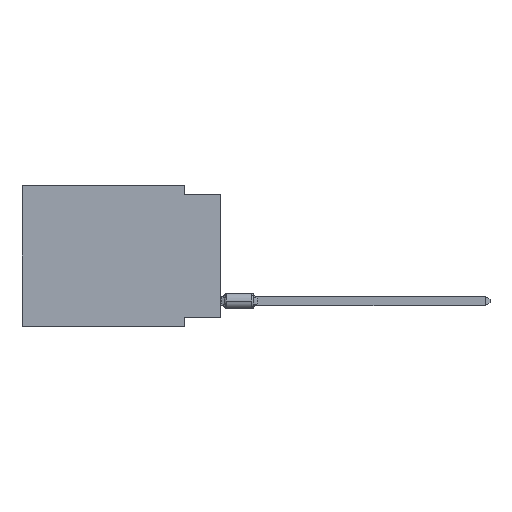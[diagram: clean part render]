
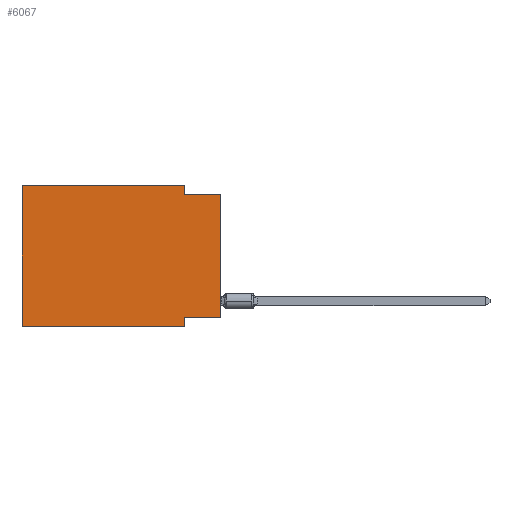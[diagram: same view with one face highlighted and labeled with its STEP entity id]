
A CAD part, left-side view. The second image highlights one B-rep face of the part: STEP entity #6067.
In plain terms, the highlighted planar face has unit normal (-1, 0, 0).
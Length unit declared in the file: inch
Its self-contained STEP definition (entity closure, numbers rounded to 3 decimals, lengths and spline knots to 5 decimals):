
#204 = VERTEX_POINT ( 'NONE', #6549 ) ;
#2309 = DIRECTION ( 'NONE',  ( 0., 0., -1. ) ) ;
#2672 = VERTEX_POINT ( 'NONE', #25112 ) ;
#3417 = VERTEX_POINT ( 'NONE', #29619 ) ;
#3538 = CARTESIAN_POINT ( 'NONE',  ( 0., 0., -0.025 ) ) ;
#3562 = VECTOR ( 'NONE', #2309, 39.37008 ) ;
#3690 = CARTESIAN_POINT ( 'NONE',  ( 0., 0., 0. ) ) ;
#3943 = CARTESIAN_POINT ( 'NONE',  ( 0., 0.1, 0. ) ) ;
#3959 = VECTOR ( 'NONE', #8955, 39.37008 ) ;
#4258 = ORIENTED_EDGE ( 'NONE', *, *, #20198, .F. ) ;
#4618 = EDGE_CURVE ( 'NONE', #204, #3417, #23734, .T. ) ;
#4672 = CARTESIAN_POINT ( 'NONE',  ( 0., 0.1, -0.39 ) ) ;
#5339 = LINE ( 'NONE', #34681, #6964 ) ;
#6067 = ADVANCED_FACE ( 'NONE', ( #21899 ), #22459, .F. ) ;
#6472 = VERTEX_POINT ( 'NONE', #13834 ) ;
#6549 = CARTESIAN_POINT ( 'NONE',  ( 0., 0.55, 0. ) ) ;
#6585 = VERTEX_POINT ( 'NONE', #14967 ) ;
#6964 = VECTOR ( 'NONE', #20259, 39.37008 ) ;
#8955 = DIRECTION ( 'NONE',  ( 0., 0., 1. ) ) ;
#9156 = DIRECTION ( 'NONE',  ( 0., -1., 0. ) ) ;
#9715 = DIRECTION ( 'NONE',  ( 0., -1., 0. ) ) ;
#9748 = VECTOR ( 'NONE', #9156, 39.37008 ) ;
#10490 = EDGE_CURVE ( 'NONE', #3417, #2672, #29848, .T. ) ;
#10832 = ORIENTED_EDGE ( 'NONE', *, *, #33181, .F. ) ;
#11297 = ORIENTED_EDGE ( 'NONE', *, *, #18778, .F. ) ;
#11999 = CARTESIAN_POINT ( 'NONE',  ( 0., 0.55, 0. ) ) ;
#12573 = LINE ( 'NONE', #3538, #19518 ) ;
#12607 = DIRECTION ( 'NONE',  ( 0., 0., -1. ) ) ;
#13574 = VECTOR ( 'NONE', #26691, 39.37008 ) ;
#13834 = CARTESIAN_POINT ( 'NONE',  ( 0., 0., -0.365 ) ) ;
#14967 = CARTESIAN_POINT ( 'NONE',  ( 0., 0.55, -0.39 ) ) ;
#15401 = LINE ( 'NONE', #35680, #36812 ) ;
#15549 = EDGE_LOOP ( 'NONE', ( #34981, #10832, #30154, #18344, #4258, #22154, #11297, #31808 ) ) ;
#17045 = CARTESIAN_POINT ( 'NONE',  ( 0., 0.1, -0.365 ) ) ;
#17069 = EDGE_CURVE ( 'NONE', #6585, #26470, #15401, .T. ) ;
#17406 = CARTESIAN_POINT ( 'NONE',  ( 0., 0.55, 0. ) ) ;
#17980 = LINE ( 'NONE', #17406, #13574 ) ;
#18344 = ORIENTED_EDGE ( 'NONE', *, *, #4618, .F. ) ;
#18778 = EDGE_CURVE ( 'NONE', #31019, #26470, #25176, .T. ) ;
#19518 = VECTOR ( 'NONE', #23936, 39.37008 ) ;
#20198 = EDGE_CURVE ( 'NONE', #6585, #204, #17980, .T. ) ;
#20259 = DIRECTION ( 'NONE',  ( 0., 1., 0. ) ) ;
#21899 = FACE_OUTER_BOUND ( 'NONE', #15549, .T. ) ;
#22090 = EDGE_CURVE ( 'NONE', #6472, #22195, #29604, .T. ) ;
#22154 = ORIENTED_EDGE ( 'NONE', *, *, #17069, .T. ) ;
#22195 = VERTEX_POINT ( 'NONE', #36598 ) ;
#22459 = PLANE ( 'NONE',  #24341 ) ;
#23734 = LINE ( 'NONE', #11999, #9748 ) ;
#23936 = DIRECTION ( 'NONE',  ( 0., -1., 0. ) ) ;
#24341 = AXIS2_PLACEMENT_3D ( 'NONE', #33463, #28519, #33837 ) ;
#25112 = CARTESIAN_POINT ( 'NONE',  ( 0., 0.1, -0.025 ) ) ;
#25176 = LINE ( 'NONE', #25354, #3562 ) ;
#25354 = CARTESIAN_POINT ( 'NONE',  ( 0., 0.1, -0.39 ) ) ;
#26470 = VERTEX_POINT ( 'NONE', #4672 ) ;
#26691 = DIRECTION ( 'NONE',  ( 0., 0., 1. ) ) ;
#28519 = DIRECTION ( 'NONE',  ( 1., 0., 0. ) ) ;
#29604 = LINE ( 'NONE', #3690, #3959 ) ;
#29619 = CARTESIAN_POINT ( 'NONE',  ( 0., 0.1, 0. ) ) ;
#29826 = VECTOR ( 'NONE', #12607, 39.37008 ) ;
#29848 = LINE ( 'NONE', #3943, #29826 ) ;
#30154 = ORIENTED_EDGE ( 'NONE', *, *, #10490, .F. ) ;
#31019 = VERTEX_POINT ( 'NONE', #17045 ) ;
#31808 = ORIENTED_EDGE ( 'NONE', *, *, #35087, .F. ) ;
#33181 = EDGE_CURVE ( 'NONE', #2672, #22195, #12573, .T. ) ;
#33463 = CARTESIAN_POINT ( 'NONE',  ( 0., 0.55, 0. ) ) ;
#33837 = DIRECTION ( 'NONE',  ( 0., 0., -1. ) ) ;
#34681 = CARTESIAN_POINT ( 'NONE',  ( 0., 0., -0.365 ) ) ;
#34981 = ORIENTED_EDGE ( 'NONE', *, *, #22090, .T. ) ;
#35087 = EDGE_CURVE ( 'NONE', #6472, #31019, #5339, .T. ) ;
#35680 = CARTESIAN_POINT ( 'NONE',  ( 0., 0.55, -0.39 ) ) ;
#36598 = CARTESIAN_POINT ( 'NONE',  ( 0., 0., -0.025 ) ) ;
#36812 = VECTOR ( 'NONE', #9715, 39.37008 ) ;
